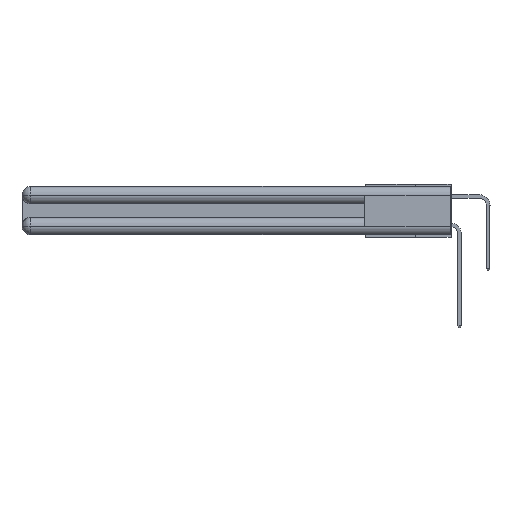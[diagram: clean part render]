
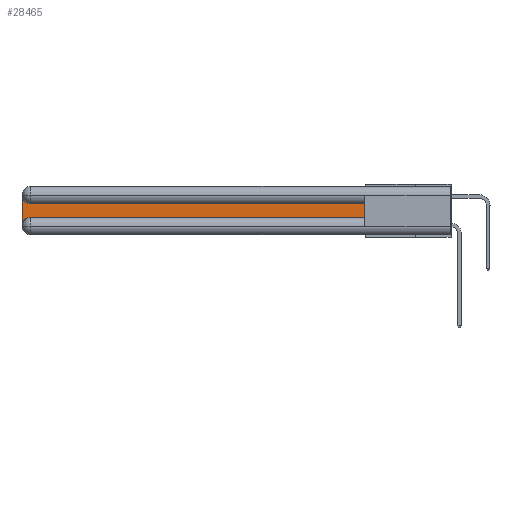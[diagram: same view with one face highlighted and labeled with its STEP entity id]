
A CAD part, left-side view. The second image highlights one B-rep face of the part: STEP entity #28465.
In plain terms, the highlighted planar face has unit normal (-1, 0, 0).
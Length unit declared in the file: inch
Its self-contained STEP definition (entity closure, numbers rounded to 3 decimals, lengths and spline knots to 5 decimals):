
#507 = DIRECTION ( 'NONE',  ( 1., 0., 0. ) ) ;
#534 = CARTESIAN_POINT ( 'NONE',  ( 0.075, 3., -0.2775 ) ) ;
#781 = CARTESIAN_POINT ( 'NONE',  ( 0.075, 3., -0.1225 ) ) ;
#991 = VERTEX_POINT ( 'NONE', #13293 ) ;
#1377 = ORIENTED_EDGE ( 'NONE', *, *, #7996, .T. ) ;
#3530 = AXIS2_PLACEMENT_3D ( 'NONE', #11682, #507, #20809 ) ;
#3700 = DIRECTION ( 'NONE',  ( 1., 0., 0. ) ) ;
#3885 = VECTOR ( 'NONE', #29717, 39.37008 ) ;
#4600 = EDGE_CURVE ( 'NONE', #35321, #25007, #15854, .T. ) ;
#5421 = AXIS2_PLACEMENT_3D ( 'NONE', #26673, #21101, #24014 ) ;
#7996 = EDGE_CURVE ( 'NONE', #28463, #24393, #16868, .T. ) ;
#8420 = CARTESIAN_POINT ( 'NONE',  ( 0.075, 0.6, -0.1225 ) ) ;
#10130 = VERTEX_POINT ( 'NONE', #8420 ) ;
#11224 = VECTOR ( 'NONE', #29686, 39.37008 ) ;
#11682 = CARTESIAN_POINT ( 'NONE',  ( 0.075, 2.94, -0.2775 ) ) ;
#12807 = CARTESIAN_POINT ( 'NONE',  ( 0.075, 3., -0.2175 ) ) ;
#13126 = AXIS2_PLACEMENT_3D ( 'NONE', #781, #3700, #15244 ) ;
#13293 = CARTESIAN_POINT ( 'NONE',  ( 0.075, 0.6, -0.2175 ) ) ;
#14662 = LINE ( 'NONE', #12807, #31459 ) ;
#15010 = CARTESIAN_POINT ( 'NONE',  ( 0.075, 2.94, -0.2175 ) ) ;
#15096 = CARTESIAN_POINT ( 'NONE',  ( 0.075, 3., -0.0625 ) ) ;
#15244 = DIRECTION ( 'NONE',  ( 0., 0., -1. ) ) ;
#15768 = VECTOR ( 'NONE', #31680, 39.37008 ) ;
#15854 = CIRCLE ( 'NONE', #5421, 0.06 ) ;
#16868 = CIRCLE ( 'NONE', #3530, 0.06 ) ;
#17098 = CARTESIAN_POINT ( 'NONE',  ( 0.075, 0.6, -0.2175 ) ) ;
#18987 = LINE ( 'NONE', #20929, #11224 ) ;
#19578 = EDGE_CURVE ( 'NONE', #24393, #991, #27111, .T. ) ;
#19652 = DIRECTION ( 'NONE',  ( 0., 0., -1. ) ) ;
#20262 = LINE ( 'NONE', #32922, #3885 ) ;
#20809 = DIRECTION ( 'NONE',  ( 0., 0., -1. ) ) ;
#20929 = CARTESIAN_POINT ( 'NONE',  ( 0.075, 0.6, -0.1225 ) ) ;
#21101 = DIRECTION ( 'NONE',  ( 1., 0., 0. ) ) ;
#22410 = CARTESIAN_POINT ( 'NONE',  ( 0.075, 2.94, -0.1225 ) ) ;
#22785 = ORIENTED_EDGE ( 'NONE', *, *, #30605, .T. ) ;
#23994 = PLANE ( 'NONE',  #13126 ) ;
#24014 = DIRECTION ( 'NONE',  ( 0., 0., -1. ) ) ;
#24393 = VERTEX_POINT ( 'NONE', #15010 ) ;
#24471 = ORIENTED_EDGE ( 'NONE', *, *, #4600, .T. ) ;
#24544 = EDGE_CURVE ( 'NONE', #991, #10130, #20262, .T. ) ;
#25007 = VERTEX_POINT ( 'NONE', #15096 ) ;
#26316 = EDGE_CURVE ( 'NONE', #25007, #28463, #14662, .T. ) ;
#26333 = EDGE_LOOP ( 'NONE', ( #22785, #24471, #35816, #1377, #33036, #28730 ) ) ;
#26673 = CARTESIAN_POINT ( 'NONE',  ( 0.075, 2.94, -0.0625 ) ) ;
#27111 = LINE ( 'NONE', #17098, #15768 ) ;
#28463 = VERTEX_POINT ( 'NONE', #534 ) ;
#28465 = ADVANCED_FACE ( 'NONE', ( #30857 ), #23994, .F. ) ;
#28730 = ORIENTED_EDGE ( 'NONE', *, *, #24544, .T. ) ;
#29686 = DIRECTION ( 'NONE',  ( 0., 1., 0. ) ) ;
#29717 = DIRECTION ( 'NONE',  ( 0., 0., 1. ) ) ;
#30605 = EDGE_CURVE ( 'NONE', #10130, #35321, #18987, .T. ) ;
#30857 = FACE_OUTER_BOUND ( 'NONE', #26333, .T. ) ;
#31459 = VECTOR ( 'NONE', #19652, 39.37008 ) ;
#31680 = DIRECTION ( 'NONE',  ( 0., -1., 0. ) ) ;
#32922 = CARTESIAN_POINT ( 'NONE',  ( 0.075, 0.6, -0.2175 ) ) ;
#33036 = ORIENTED_EDGE ( 'NONE', *, *, #19578, .T. ) ;
#35321 = VERTEX_POINT ( 'NONE', #22410 ) ;
#35816 = ORIENTED_EDGE ( 'NONE', *, *, #26316, .T. ) ;
